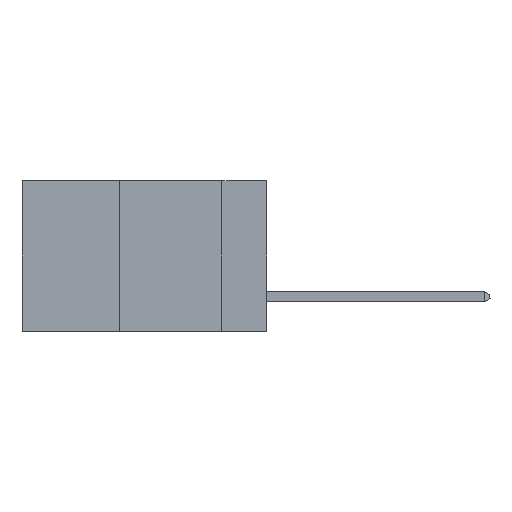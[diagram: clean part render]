
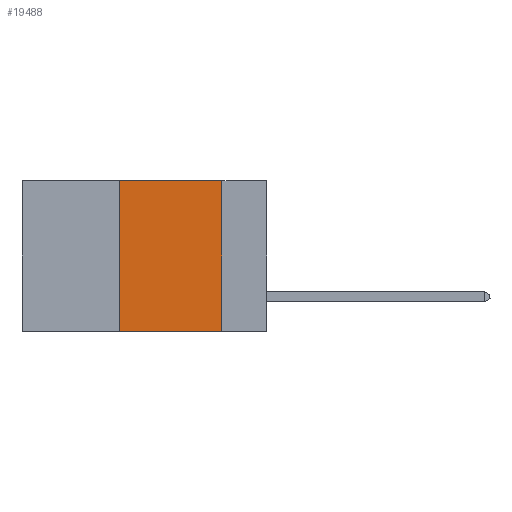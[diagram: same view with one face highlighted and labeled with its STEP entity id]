
A CAD part, left-side view. The second image highlights one B-rep face of the part: STEP entity #19488.
In plain terms, the highlighted planar face has unit normal (-1, 0, 0).
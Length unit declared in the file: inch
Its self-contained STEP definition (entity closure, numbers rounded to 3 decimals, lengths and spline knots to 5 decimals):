
#115 = DIRECTION ( 'NONE',  ( 0., 0., -1. ) ) ;
#937 = LINE ( 'NONE', #10197, #15394 ) ;
#1242 = FACE_OUTER_BOUND ( 'NONE', #2828, .T. ) ;
#2828 = EDGE_LOOP ( 'NONE', ( #10376, #11900, #17537, #23608 ) ) ;
#3177 = CARTESIAN_POINT ( 'NONE',  ( 0., 0.11, 0. ) ) ;
#3280 = VERTEX_POINT ( 'NONE', #24208 ) ;
#5724 = EDGE_CURVE ( 'NONE', #3280, #10055, #10575, .T. ) ;
#5765 = CARTESIAN_POINT ( 'NONE',  ( 0., 0.11, 0. ) ) ;
#6338 = DIRECTION ( 'NONE',  ( 0., 0., -1. ) ) ;
#7008 = VECTOR ( 'NONE', #16179, 39.37008 ) ;
#8624 = CARTESIAN_POINT ( 'NONE',  ( 0., 0.6, 0. ) ) ;
#9031 = EDGE_CURVE ( 'NONE', #23703, #22307, #12209, .T. ) ;
#10055 = VERTEX_POINT ( 'NONE', #12864 ) ;
#10152 = CARTESIAN_POINT ( 'NONE',  ( 0., 0.36, 0. ) ) ;
#10197 = CARTESIAN_POINT ( 'NONE',  ( 0., 0.6, -0.37 ) ) ;
#10376 = ORIENTED_EDGE ( 'NONE', *, *, #9031, .F. ) ;
#10575 = LINE ( 'NONE', #10152, #11792 ) ;
#11792 = VECTOR ( 'NONE', #21466, 39.37008 ) ;
#11900 = ORIENTED_EDGE ( 'NONE', *, *, #14265, .F. ) ;
#12209 = LINE ( 'NONE', #5765, #21617 ) ;
#12864 = CARTESIAN_POINT ( 'NONE',  ( 0., 0.36, 0. ) ) ;
#13894 = PLANE ( 'NONE',  #15041 ) ;
#14150 = CARTESIAN_POINT ( 'NONE',  ( 0., 0.11, -0.37 ) ) ;
#14265 = EDGE_CURVE ( 'NONE', #10055, #23703, #16467, .T. ) ;
#15041 = AXIS2_PLACEMENT_3D ( 'NONE', #15771, #17669, #6338 ) ;
#15394 = VECTOR ( 'NONE', #23337, 39.37008 ) ;
#15771 = CARTESIAN_POINT ( 'NONE',  ( 0., 0.6, 0. ) ) ;
#16179 = DIRECTION ( 'NONE',  ( 0., -1., 0. ) ) ;
#16467 = LINE ( 'NONE', #8624, #7008 ) ;
#17537 = ORIENTED_EDGE ( 'NONE', *, *, #5724, .F. ) ;
#17669 = DIRECTION ( 'NONE',  ( 1., 0., 0. ) ) ;
#17956 = EDGE_CURVE ( 'NONE', #3280, #22307, #937, .T. ) ;
#19488 = ADVANCED_FACE ( 'NONE', ( #1242 ), #13894, .F. ) ;
#21466 = DIRECTION ( 'NONE',  ( 0., 0., 1. ) ) ;
#21617 = VECTOR ( 'NONE', #115, 39.37008 ) ;
#22307 = VERTEX_POINT ( 'NONE', #14150 ) ;
#23337 = DIRECTION ( 'NONE',  ( 0., -1., 0. ) ) ;
#23608 = ORIENTED_EDGE ( 'NONE', *, *, #17956, .T. ) ;
#23703 = VERTEX_POINT ( 'NONE', #3177 ) ;
#24208 = CARTESIAN_POINT ( 'NONE',  ( 0., 0.36, -0.37 ) ) ;
